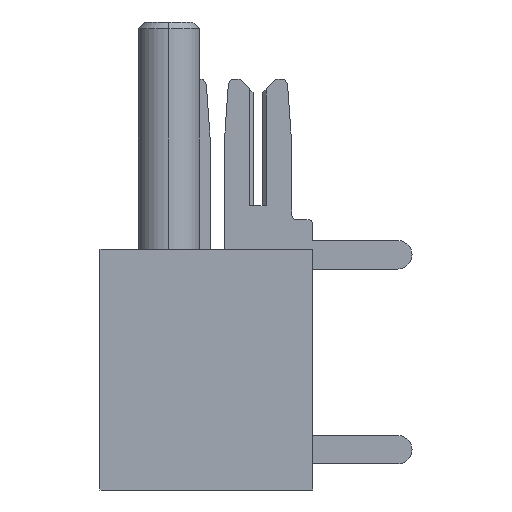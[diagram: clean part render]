
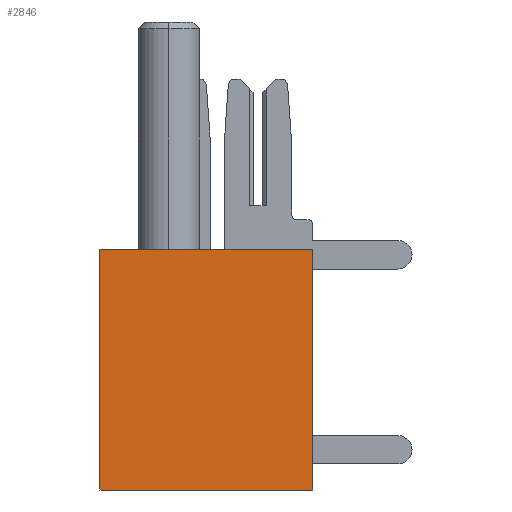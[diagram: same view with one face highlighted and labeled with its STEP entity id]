
A CAD part, left-side view. The second image highlights one B-rep face of the part: STEP entity #2846.
In plain terms, the highlighted planar face has unit normal (-1, 0, 0).
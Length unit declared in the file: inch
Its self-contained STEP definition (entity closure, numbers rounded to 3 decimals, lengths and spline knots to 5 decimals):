
#32 = DIRECTION ( 'NONE',  ( 0., 0., 1. ) ) ;
#241 = CARTESIAN_POINT ( 'NONE',  ( 0., 0., -0.37 ) ) ;
#400 = CARTESIAN_POINT ( 'NONE',  ( 0., 0., -0.37 ) ) ;
#452 = DIRECTION ( 'NONE',  ( 0., 0., 1. ) ) ;
#710 = EDGE_CURVE ( 'NONE', #4975, #2489, #5445, .T. ) ;
#1170 = CARTESIAN_POINT ( 'NONE',  ( 0., 0.327, -0.37 ) ) ;
#1211 = VECTOR ( 'NONE', #3972, 39.37008 ) ;
#1339 = EDGE_CURVE ( 'NONE', #2489, #1515, #4490, .T. ) ;
#1515 = VERTEX_POINT ( 'NONE', #6038 ) ;
#2489 = VERTEX_POINT ( 'NONE', #6165 ) ;
#2708 = DIRECTION ( 'NONE',  ( 0., -1., 0. ) ) ;
#2811 = PLANE ( 'NONE',  #6185 ) ;
#2846 = ADVANCED_FACE ( 'NONE', ( #6572 ), #2811, .T. ) ;
#2864 = DIRECTION ( 'NONE',  ( -1., 0., 0. ) ) ;
#3166 = EDGE_LOOP ( 'NONE', ( #4829, #3255, #4458, #7637 ) ) ;
#3255 = ORIENTED_EDGE ( 'NONE', *, *, #5065, .F. ) ;
#3532 = VERTEX_POINT ( 'NONE', #6549 ) ;
#3972 = DIRECTION ( 'NONE',  ( 0., -1., 0. ) ) ;
#4458 = ORIENTED_EDGE ( 'NONE', *, *, #710, .T. ) ;
#4490 = LINE ( 'NONE', #241, #6575 ) ;
#4829 = ORIENTED_EDGE ( 'NONE', *, *, #6139, .F. ) ;
#4975 = VERTEX_POINT ( 'NONE', #1170 ) ;
#5065 = EDGE_CURVE ( 'NONE', #4975, #3532, #6393, .T. ) ;
#5124 = DIRECTION ( 'NONE',  ( 0., 0., 1. ) ) ;
#5445 = LINE ( 'NONE', #6260, #5740 ) ;
#5451 = CARTESIAN_POINT ( 'NONE',  ( 0., 0.327, -0.37 ) ) ;
#5740 = VECTOR ( 'NONE', #2708, 39.37008 ) ;
#6038 = CARTESIAN_POINT ( 'NONE',  ( 0., 0., 0. ) ) ;
#6139 = EDGE_CURVE ( 'NONE', #3532, #1515, #6206, .T. ) ;
#6165 = CARTESIAN_POINT ( 'NONE',  ( 0., 0., -0.37 ) ) ;
#6185 = AXIS2_PLACEMENT_3D ( 'NONE', #400, #2864, #452 ) ;
#6206 = LINE ( 'NONE', #7603, #1211 ) ;
#6260 = CARTESIAN_POINT ( 'NONE',  ( 0., 0., -0.37 ) ) ;
#6393 = LINE ( 'NONE', #5451, #7500 ) ;
#6549 = CARTESIAN_POINT ( 'NONE',  ( 0., 0.327, 0. ) ) ;
#6572 = FACE_OUTER_BOUND ( 'NONE', #3166, .T. ) ;
#6575 = VECTOR ( 'NONE', #5124, 39.37008 ) ;
#7500 = VECTOR ( 'NONE', #32, 39.37008 ) ;
#7603 = CARTESIAN_POINT ( 'NONE',  ( 0., 0., 0. ) ) ;
#7637 = ORIENTED_EDGE ( 'NONE', *, *, #1339, .T. ) ;
